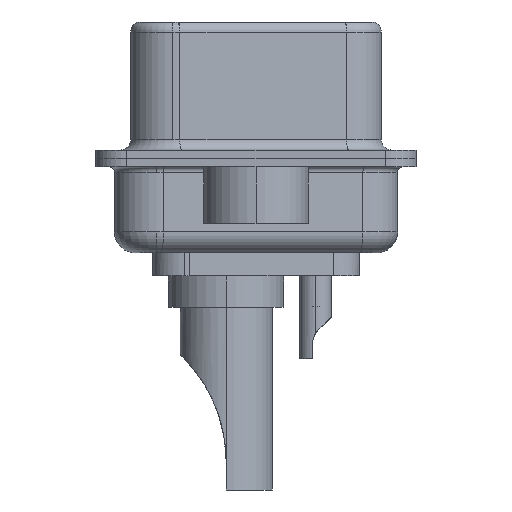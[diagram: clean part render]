
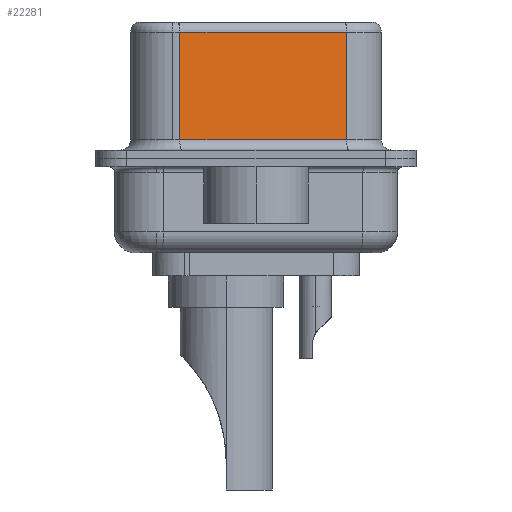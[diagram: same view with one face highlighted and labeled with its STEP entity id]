
A CAD part, left-side view. The second image highlights one B-rep face of the part: STEP entity #22281.
In plain terms, the highlighted planar face has unit normal (-0.985, -0.174, 0).
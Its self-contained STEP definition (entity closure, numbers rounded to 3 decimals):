
#1193 = VERTEX_POINT ( 'NONE', #3730 ) ;
#1475 = DIRECTION ( 'NONE',  ( -0.174, 0.985, 0. ) ) ;
#2398 = DIRECTION ( 'NONE',  ( 0.174, -0.985, 0. ) ) ;
#3231 = EDGE_CURVE ( 'NONE', #12453, #22792, #4022, .T. ) ;
#3730 = CARTESIAN_POINT ( 'NONE',  ( 3.73, 3.628, 6.02 ) ) ;
#4022 = LINE ( 'NONE', #7764, #26312 ) ;
#4195 = DIRECTION ( 'NONE',  ( 0., 0., -1. ) ) ;
#4908 = AXIS2_PLACEMENT_3D ( 'NONE', #9309, #24113, #11397 ) ;
#5520 = CARTESIAN_POINT ( 'NONE',  ( 5.132, -4.322, 6.02 ) ) ;
#7110 = DIRECTION ( 'NONE',  ( 0., 0., -1. ) ) ;
#7764 = CARTESIAN_POINT ( 'NONE',  ( 5.132, -4.322, 6.52 ) ) ;
#9211 = CARTESIAN_POINT ( 'NONE',  ( 5.132, -4.322, 0.9 ) ) ;
#9309 = CARTESIAN_POINT ( 'NONE',  ( 5.132, -4.322, 6.52 ) ) ;
#9476 = EDGE_CURVE ( 'NONE', #12453, #1193, #26955, .T. ) ;
#9528 = ORIENTED_EDGE ( 'NONE', *, *, #26216, .T. ) ;
#10559 = CARTESIAN_POINT ( 'NONE',  ( 5.132, -4.322, 0.9 ) ) ;
#11397 = DIRECTION ( 'NONE',  ( -0.174, 0.985, 0. ) ) ;
#12446 = CARTESIAN_POINT ( 'NONE',  ( 3.73, 3.628, 6.52 ) ) ;
#12453 = VERTEX_POINT ( 'NONE', #23160 ) ;
#12671 = CARTESIAN_POINT ( 'NONE',  ( 3.73, 3.628, 0.9 ) ) ;
#14586 = VERTEX_POINT ( 'NONE', #12671 ) ;
#15507 = EDGE_LOOP ( 'NONE', ( #17744, #25580, #20030, #9528 ) ) ;
#16088 = FACE_OUTER_BOUND ( 'NONE', #15507, .T. ) ;
#17744 = ORIENTED_EDGE ( 'NONE', *, *, #3231, .F. ) ;
#17882 = VECTOR ( 'NONE', #2398, 1000. ) ;
#20030 = ORIENTED_EDGE ( 'NONE', *, *, #21135, .T. ) ;
#20133 = VECTOR ( 'NONE', #4195, 1000. ) ;
#20791 = LINE ( 'NONE', #12446, #20133 ) ;
#21135 = EDGE_CURVE ( 'NONE', #1193, #14586, #20791, .T. ) ;
#21412 = VECTOR ( 'NONE', #1475, 1000. ) ;
#21988 = PLANE ( 'NONE',  #4908 ) ;
#22281 = ADVANCED_FACE ( 'NONE', ( #16088 ), #21988, .F. ) ;
#22792 = VERTEX_POINT ( 'NONE', #9211 ) ;
#23160 = CARTESIAN_POINT ( 'NONE',  ( 5.132, -4.322, 6.02 ) ) ;
#23553 = LINE ( 'NONE', #10559, #17882 ) ;
#24113 = DIRECTION ( 'NONE',  ( 0.985, 0.174, 0. ) ) ;
#25580 = ORIENTED_EDGE ( 'NONE', *, *, #9476, .T. ) ;
#26216 = EDGE_CURVE ( 'NONE', #14586, #22792, #23553, .T. ) ;
#26312 = VECTOR ( 'NONE', #7110, 1000. ) ;
#26955 = LINE ( 'NONE', #5520, #21412 ) ;
